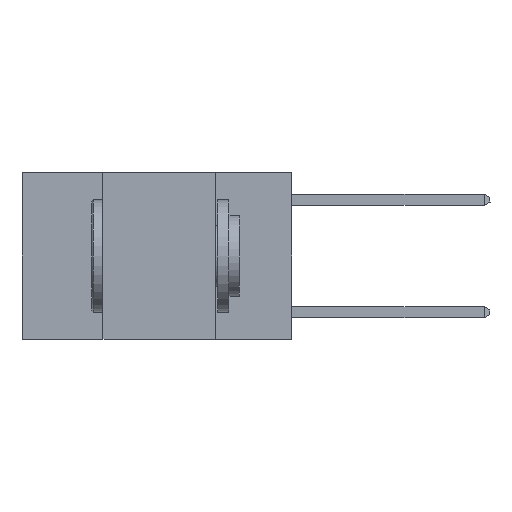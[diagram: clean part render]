
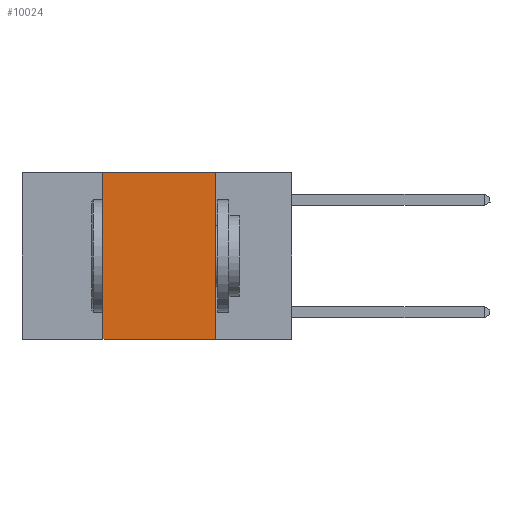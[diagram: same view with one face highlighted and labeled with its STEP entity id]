
A CAD part, left-side view. The second image highlights one B-rep face of the part: STEP entity #10024.
In plain terms, the highlighted planar face has unit normal (-1, 0, 0).
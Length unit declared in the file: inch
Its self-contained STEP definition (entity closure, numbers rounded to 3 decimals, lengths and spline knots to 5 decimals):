
#311 = EDGE_CURVE ( 'NONE', #8825, #12068, #7227, .T. ) ;
#364 = EDGE_CURVE ( 'NONE', #11008, #9614, #2608, .T. ) ;
#455 = DIRECTION ( 'NONE',  ( 0., 0., 1. ) ) ;
#754 = EDGE_CURVE ( 'NONE', #12068, #11008, #15599, .T. ) ;
#1231 = PLANE ( 'NONE',  #5293 ) ;
#1506 = FACE_OUTER_BOUND ( 'NONE', #1512, .T. ) ;
#1512 = EDGE_LOOP ( 'NONE', ( #3584, #6937, #10341, #13664 ) ) ;
#1910 = CARTESIAN_POINT ( 'NONE',  ( 0., 0.42, -0.37 ) ) ;
#2608 = LINE ( 'NONE', #3785, #9036 ) ;
#3346 = EDGE_CURVE ( 'NONE', #8825, #9614, #10923, .T. ) ;
#3584 = ORIENTED_EDGE ( 'NONE', *, *, #364, .F. ) ;
#3785 = CARTESIAN_POINT ( 'NONE',  ( 0., 0.17, 0. ) ) ;
#5293 = AXIS2_PLACEMENT_3D ( 'NONE', #15477, #7883, #16710 ) ;
#5775 = DIRECTION ( 'NONE',  ( 0., 0., -1. ) ) ;
#6877 = CARTESIAN_POINT ( 'NONE',  ( 0., 0.17, 0. ) ) ;
#6937 = ORIENTED_EDGE ( 'NONE', *, *, #754, .F. ) ;
#6942 = CARTESIAN_POINT ( 'NONE',  ( 0., 0.6, 0. ) ) ;
#7037 = DIRECTION ( 'NONE',  ( 0., -1., 0. ) ) ;
#7227 = LINE ( 'NONE', #9165, #13557 ) ;
#7231 = DIRECTION ( 'NONE',  ( 0., -1., 0. ) ) ;
#7487 = CARTESIAN_POINT ( 'NONE',  ( 0., 0.42, 0. ) ) ;
#7883 = DIRECTION ( 'NONE',  ( 1., 0., 0. ) ) ;
#8463 = VECTOR ( 'NONE', #7037, 39.37008 ) ;
#8825 = VERTEX_POINT ( 'NONE', #1910 ) ;
#9036 = VECTOR ( 'NONE', #5775, 39.37008 ) ;
#9165 = CARTESIAN_POINT ( 'NONE',  ( 0., 0.42, 0. ) ) ;
#9614 = VERTEX_POINT ( 'NONE', #11030 ) ;
#10024 = ADVANCED_FACE ( 'NONE', ( #1506 ), #1231, .F. ) ;
#10341 = ORIENTED_EDGE ( 'NONE', *, *, #311, .F. ) ;
#10923 = LINE ( 'NONE', #11017, #11302 ) ;
#11008 = VERTEX_POINT ( 'NONE', #6877 ) ;
#11017 = CARTESIAN_POINT ( 'NONE',  ( 0., 0.6, -0.37 ) ) ;
#11030 = CARTESIAN_POINT ( 'NONE',  ( 0., 0.17, -0.37 ) ) ;
#11302 = VECTOR ( 'NONE', #7231, 39.37008 ) ;
#12068 = VERTEX_POINT ( 'NONE', #7487 ) ;
#13557 = VECTOR ( 'NONE', #455, 39.37008 ) ;
#13664 = ORIENTED_EDGE ( 'NONE', *, *, #3346, .T. ) ;
#15477 = CARTESIAN_POINT ( 'NONE',  ( 0., 0.6, 0. ) ) ;
#15599 = LINE ( 'NONE', #6942, #8463 ) ;
#16710 = DIRECTION ( 'NONE',  ( 0., 0., -1. ) ) ;
